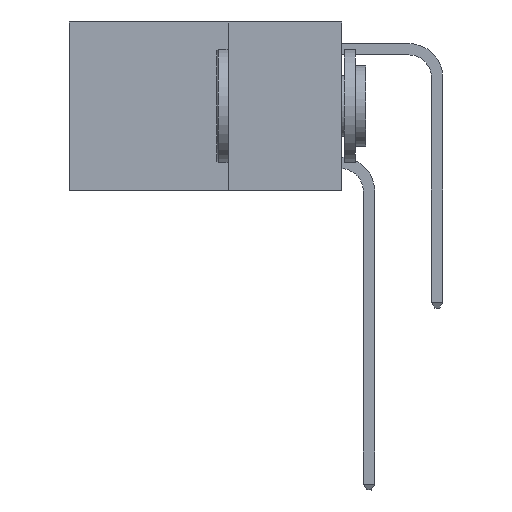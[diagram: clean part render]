
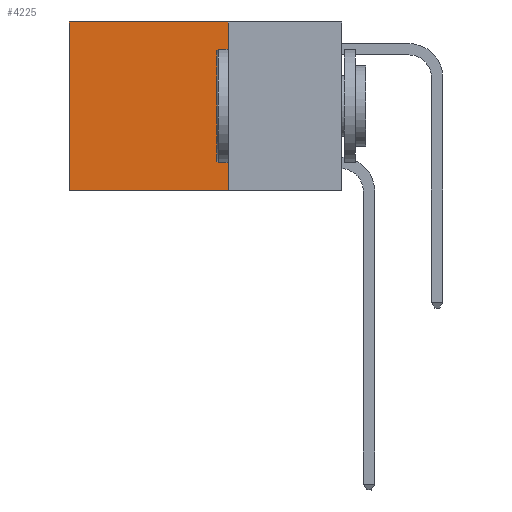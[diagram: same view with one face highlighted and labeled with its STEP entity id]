
A CAD part, left-side view. The second image highlights one B-rep face of the part: STEP entity #4225.
In plain terms, the highlighted planar face has unit normal (-1, 0, 0).
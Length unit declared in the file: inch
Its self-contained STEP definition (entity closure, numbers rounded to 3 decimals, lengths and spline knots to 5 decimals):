
#1097 = EDGE_CURVE ( 'NONE', #9835, #18222, #8021, .T. ) ;
#1299 = ORIENTED_EDGE ( 'NONE', *, *, #15090, .F. ) ;
#3980 = VECTOR ( 'NONE', #4542, 39.37008 ) ;
#4225 = ADVANCED_FACE ( 'NONE', ( #13902 ), #6233, .F. ) ;
#4542 = DIRECTION ( 'NONE',  ( 0., 0., -1. ) ) ;
#5066 = AXIS2_PLACEMENT_3D ( 'NONE', #15844, #21563, #19606 ) ;
#5763 = VERTEX_POINT ( 'NONE', #20287 ) ;
#6217 = DIRECTION ( 'NONE',  ( 0., 0., -1. ) ) ;
#6233 = PLANE ( 'NONE',  #5066 ) ;
#6367 = LINE ( 'NONE', #8439, #3980 ) ;
#7869 = ORIENTED_EDGE ( 'NONE', *, *, #1097, .T. ) ;
#7902 = CARTESIAN_POINT ( 'NONE',  ( 0.2625, 0.6, 0. ) ) ;
#8021 = LINE ( 'NONE', #7902, #23464 ) ;
#8439 = CARTESIAN_POINT ( 'NONE',  ( 0.2625, 0.25, 0. ) ) ;
#9835 = VERTEX_POINT ( 'NONE', #10906 ) ;
#10906 = CARTESIAN_POINT ( 'NONE',  ( 0.2625, 0.6, 0. ) ) ;
#11205 = DIRECTION ( 'NONE',  ( 0., 1., 0. ) ) ;
#12863 = CARTESIAN_POINT ( 'NONE',  ( 0.2625, 0.25, 0. ) ) ;
#13902 = FACE_OUTER_BOUND ( 'NONE', #17711, .T. ) ;
#15090 = EDGE_CURVE ( 'NONE', #23158, #5763, #6367, .T. ) ;
#15844 = CARTESIAN_POINT ( 'NONE',  ( 0.2625, 0.25, 0. ) ) ;
#16677 = CARTESIAN_POINT ( 'NONE',  ( 0.2625, 0.25, -0.37 ) ) ;
#17711 = EDGE_LOOP ( 'NONE', ( #7869, #24645, #1299, #23090 ) ) ;
#18222 = VERTEX_POINT ( 'NONE', #24260 ) ;
#19490 = LINE ( 'NONE', #21691, #22175 ) ;
#19606 = DIRECTION ( 'NONE',  ( 0., 0., -1. ) ) ;
#20186 = LINE ( 'NONE', #16677, #23457 ) ;
#20287 = CARTESIAN_POINT ( 'NONE',  ( 0.2625, 0.25, -0.37 ) ) ;
#21563 = DIRECTION ( 'NONE',  ( 1., 0., 0. ) ) ;
#21691 = CARTESIAN_POINT ( 'NONE',  ( 0.2625, 0.25, 0. ) ) ;
#22175 = VECTOR ( 'NONE', #11205, 39.37008 ) ;
#22267 = DIRECTION ( 'NONE',  ( 0., 1., 0. ) ) ;
#22777 = EDGE_CURVE ( 'NONE', #5763, #18222, #20186, .T. ) ;
#23090 = ORIENTED_EDGE ( 'NONE', *, *, #23863, .T. ) ;
#23158 = VERTEX_POINT ( 'NONE', #12863 ) ;
#23457 = VECTOR ( 'NONE', #22267, 39.37008 ) ;
#23464 = VECTOR ( 'NONE', #6217, 39.37008 ) ;
#23863 = EDGE_CURVE ( 'NONE', #23158, #9835, #19490, .T. ) ;
#24260 = CARTESIAN_POINT ( 'NONE',  ( 0.2625, 0.6, -0.37 ) ) ;
#24645 = ORIENTED_EDGE ( 'NONE', *, *, #22777, .F. ) ;
